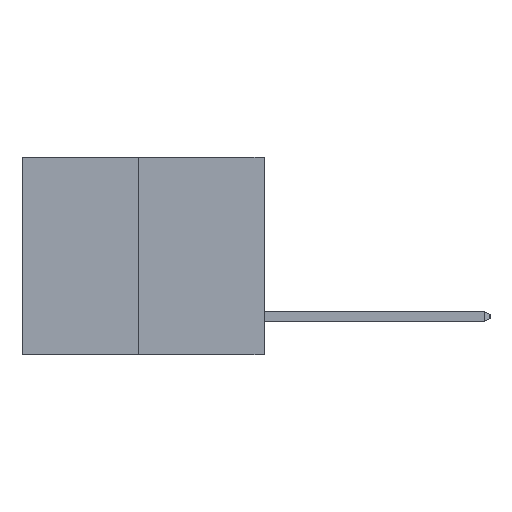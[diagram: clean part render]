
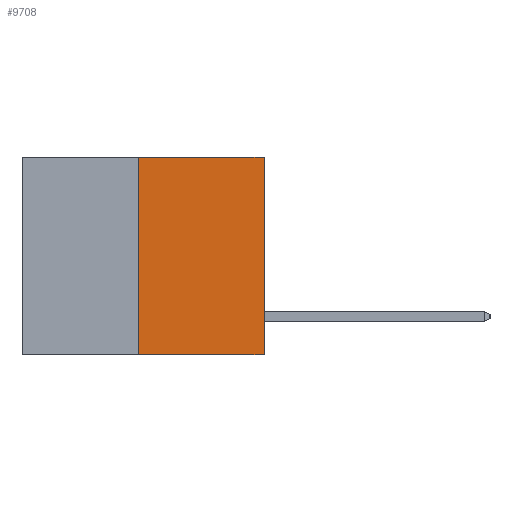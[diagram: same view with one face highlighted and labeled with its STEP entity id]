
A CAD part, left-side view. The second image highlights one B-rep face of the part: STEP entity #9708.
In plain terms, the highlighted planar face has unit normal (-1, 0, 0).
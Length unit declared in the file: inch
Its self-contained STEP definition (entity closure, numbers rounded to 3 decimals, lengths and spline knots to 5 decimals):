
#177 = VERTEX_POINT ( 'NONE', #8642 ) ;
#364 = CARTESIAN_POINT ( 'NONE',  ( 0., 0., -0.49 ) ) ;
#1005 = CARTESIAN_POINT ( 'NONE',  ( 0., 0., 0. ) ) ;
#1179 = VECTOR ( 'NONE', #3640, 39.37008 ) ;
#1805 = CARTESIAN_POINT ( 'NONE',  ( 0., 0.6, -0.49 ) ) ;
#1993 = ORIENTED_EDGE ( 'NONE', *, *, #7067, .T. ) ;
#2090 = FACE_OUTER_BOUND ( 'NONE', #6010, .T. ) ;
#2302 = VECTOR ( 'NONE', #3931, 39.37008 ) ;
#2432 = VECTOR ( 'NONE', #6544, 39.37008 ) ;
#2731 = ORIENTED_EDGE ( 'NONE', *, *, #9866, .F. ) ;
#3606 = LINE ( 'NONE', #1805, #1179 ) ;
#3640 = DIRECTION ( 'NONE',  ( 0., -1., 0. ) ) ;
#3688 = CARTESIAN_POINT ( 'NONE',  ( 0., 0.312, -0.49 ) ) ;
#3931 = DIRECTION ( 'NONE',  ( 0., -1., 0. ) ) ;
#3993 = VERTEX_POINT ( 'NONE', #1005 ) ;
#4754 = LINE ( 'NONE', #9471, #2302 ) ;
#5597 = LINE ( 'NONE', #5633, #2432 ) ;
#5633 = CARTESIAN_POINT ( 'NONE',  ( 0., 0., 0. ) ) ;
#5809 = VECTOR ( 'NONE', #6071, 39.37008 ) ;
#5938 = EDGE_CURVE ( 'NONE', #177, #3993, #4754, .T. ) ;
#6010 = EDGE_LOOP ( 'NONE', ( #2731, #6574, #1993, #7990 ) ) ;
#6071 = DIRECTION ( 'NONE',  ( 0., 0., 1. ) ) ;
#6544 = DIRECTION ( 'NONE',  ( 0., 0., 1. ) ) ;
#6574 = ORIENTED_EDGE ( 'NONE', *, *, #6632, .T. ) ;
#6632 = EDGE_CURVE ( 'NONE', #8701, #8900, #3606, .T. ) ;
#6733 = PLANE ( 'NONE',  #7885 ) ;
#7067 = EDGE_CURVE ( 'NONE', #8900, #3993, #5597, .T. ) ;
#7782 = DIRECTION ( 'NONE',  ( 1., 0., 0. ) ) ;
#7885 = AXIS2_PLACEMENT_3D ( 'NONE', #11271, #7782, #9580 ) ;
#7990 = ORIENTED_EDGE ( 'NONE', *, *, #5938, .F. ) ;
#8642 = CARTESIAN_POINT ( 'NONE',  ( 0., 0.312, 0. ) ) ;
#8701 = VERTEX_POINT ( 'NONE', #3688 ) ;
#8900 = VERTEX_POINT ( 'NONE', #364 ) ;
#9471 = CARTESIAN_POINT ( 'NONE',  ( 0., 0.6, 0. ) ) ;
#9580 = DIRECTION ( 'NONE',  ( 0., 0., -1. ) ) ;
#9708 = ADVANCED_FACE ( 'NONE', ( #2090 ), #6733, .F. ) ;
#9866 = EDGE_CURVE ( 'NONE', #8701, #177, #10463, .T. ) ;
#10463 = LINE ( 'NONE', #11672, #5809 ) ;
#11271 = CARTESIAN_POINT ( 'NONE',  ( 0., 0.6, 0. ) ) ;
#11672 = CARTESIAN_POINT ( 'NONE',  ( 0., 0.312, -0.49 ) ) ;
